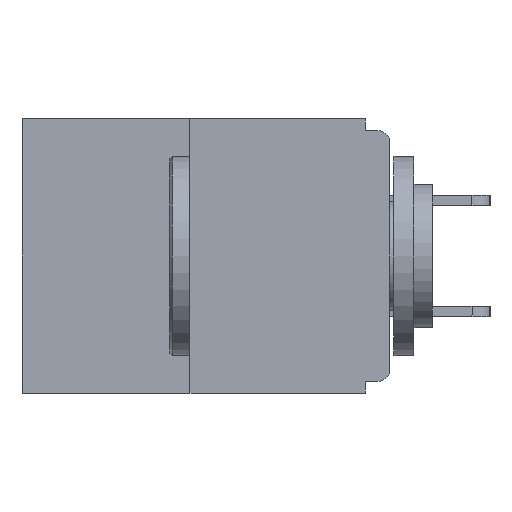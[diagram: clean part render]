
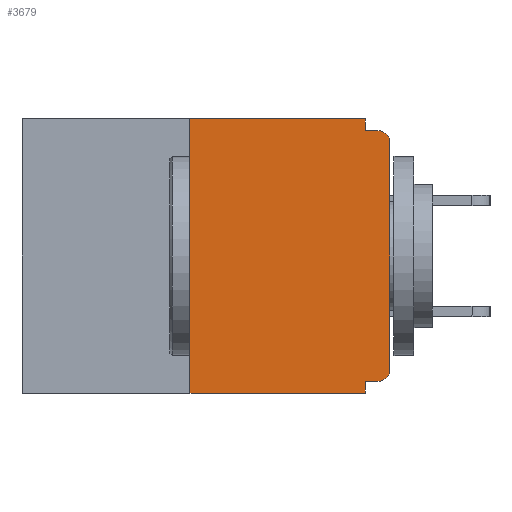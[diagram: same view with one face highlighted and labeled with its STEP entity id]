
A CAD part, left-side view. The second image highlights one B-rep face of the part: STEP entity #3679.
In plain terms, the highlighted planar face has unit normal (-1, 0, 0).
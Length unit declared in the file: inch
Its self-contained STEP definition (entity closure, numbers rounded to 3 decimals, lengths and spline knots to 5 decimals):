
#695 = CARTESIAN_POINT ( 'NONE',  ( 0., 0.031, 0. ) ) ;
#1478 = CARTESIAN_POINT ( 'NONE',  ( 0., 0.015, -0.313 ) ) ;
#1876 = ORIENTED_EDGE ( 'NONE', *, *, #5647, .F. ) ;
#1942 = CARTESIAN_POINT ( 'NONE',  ( 0., 0.46, 0. ) ) ;
#2201 = LINE ( 'NONE', #28071, #18874 ) ;
#2352 = CARTESIAN_POINT ( 'NONE',  ( 0., 0.015, -0.03 ) ) ;
#2702 = EDGE_CURVE ( 'NONE', #18080, #23388, #2201, .T. ) ;
#2946 = EDGE_LOOP ( 'NONE', ( #4588, #20163, #25656, #21828, #23723, #16641, #4883, #20448, #10286, #1876 ) ) ;
#3013 = CARTESIAN_POINT ( 'NONE',  ( 0., 0.031, -0.343 ) ) ;
#3679 = ADVANCED_FACE ( 'NONE', ( #6558 ), #10366, .F. ) ;
#3862 = CARTESIAN_POINT ( 'NONE',  ( 0., 0., -0.03 ) ) ;
#3897 = LINE ( 'NONE', #695, #11730 ) ;
#3924 = CARTESIAN_POINT ( 'NONE',  ( 0., 0.031, -0.015 ) ) ;
#4588 = ORIENTED_EDGE ( 'NONE', *, *, #27016, .F. ) ;
#4691 = DIRECTION ( 'NONE',  ( 0., 0., 1. ) ) ;
#4883 = ORIENTED_EDGE ( 'NONE', *, *, #10974, .T. ) ;
#5071 = LINE ( 'NONE', #19038, #19050 ) ;
#5340 = EDGE_CURVE ( 'NONE', #21721, #23388, #13786, .T. ) ;
#5486 = VERTEX_POINT ( 'NONE', #6380 ) ;
#5647 = EDGE_CURVE ( 'NONE', #19507, #10311, #3897, .T. ) ;
#6380 = CARTESIAN_POINT ( 'NONE',  ( 0., 0., -0.313 ) ) ;
#6484 = DIRECTION ( 'NONE',  ( 0., -1., 0. ) ) ;
#6558 = FACE_OUTER_BOUND ( 'NONE', #2946, .T. ) ;
#6775 = EDGE_CURVE ( 'NONE', #10311, #25107, #17444, .T. ) ;
#7209 = VECTOR ( 'NONE', #4691, 39.37008 ) ;
#7794 = DIRECTION ( 'NONE',  ( 0., 0., -1. ) ) ;
#7961 = LINE ( 'NONE', #1942, #25646 ) ;
#7981 = AXIS2_PLACEMENT_3D ( 'NONE', #2352, #28174, #24644 ) ;
#8359 = EDGE_CURVE ( 'NONE', #24460, #21721, #13274, .T. ) ;
#9212 = VERTEX_POINT ( 'NONE', #21654 ) ;
#9595 = CARTESIAN_POINT ( 'NONE',  ( 0., 0.031, 0. ) ) ;
#10286 = ORIENTED_EDGE ( 'NONE', *, *, #6775, .F. ) ;
#10311 = VERTEX_POINT ( 'NONE', #3924 ) ;
#10366 = PLANE ( 'NONE',  #26236 ) ;
#10974 = EDGE_CURVE ( 'NONE', #5486, #12482, #5071, .T. ) ;
#11730 = VECTOR ( 'NONE', #18114, 39.37008 ) ;
#12182 = CARTESIAN_POINT ( 'NONE',  ( 0., 0.46, 0. ) ) ;
#12482 = VERTEX_POINT ( 'NONE', #3862 ) ;
#12655 = DIRECTION ( 'NONE',  ( 0., 0., 1. ) ) ;
#13274 = LINE ( 'NONE', #15088, #23460 ) ;
#13507 = CARTESIAN_POINT ( 'NONE',  ( 0., 0.015, -0.328 ) ) ;
#13786 = LINE ( 'NONE', #20881, #24648 ) ;
#15088 = CARTESIAN_POINT ( 'NONE',  ( 0., 0., -0.328 ) ) ;
#15745 = VECTOR ( 'NONE', #25598, 39.37008 ) ;
#15865 = EDGE_CURVE ( 'NONE', #18080, #9212, #18818, .T. ) ;
#16104 = EDGE_CURVE ( 'NONE', #12482, #25107, #19480, .T. ) ;
#16430 = EDGE_CURVE ( 'NONE', #24460, #5486, #21475, .T. ) ;
#16641 = ORIENTED_EDGE ( 'NONE', *, *, #16430, .T. ) ;
#16699 = DIRECTION ( 'NONE',  ( -1., 0., 0. ) ) ;
#17444 = LINE ( 'NONE', #25686, #15745 ) ;
#18080 = VERTEX_POINT ( 'NONE', #27196 ) ;
#18114 = DIRECTION ( 'NONE',  ( 0., 0., -1. ) ) ;
#18667 = CARTESIAN_POINT ( 'NONE',  ( 0., 0.031, -0.328 ) ) ;
#18818 = LINE ( 'NONE', #19643, #7209 ) ;
#18874 = VECTOR ( 'NONE', #6484, 39.37008 ) ;
#19038 = CARTESIAN_POINT ( 'NONE',  ( 0., 0., 0. ) ) ;
#19050 = VECTOR ( 'NONE', #12655, 39.37008 ) ;
#19140 = AXIS2_PLACEMENT_3D ( 'NONE', #1478, #16699, #25392 ) ;
#19480 = CIRCLE ( 'NONE', #7981, 0.015 ) ;
#19492 = DIRECTION ( 'NONE',  ( 0., 1., 0. ) ) ;
#19507 = VERTEX_POINT ( 'NONE', #9595 ) ;
#19643 = CARTESIAN_POINT ( 'NONE',  ( 0., 0.25, 0. ) ) ;
#20163 = ORIENTED_EDGE ( 'NONE', *, *, #15865, .F. ) ;
#20448 = ORIENTED_EDGE ( 'NONE', *, *, #16104, .T. ) ;
#20881 = CARTESIAN_POINT ( 'NONE',  ( 0., 0.031, -0.343 ) ) ;
#21475 = CIRCLE ( 'NONE', #19140, 0.015 ) ;
#21654 = CARTESIAN_POINT ( 'NONE',  ( 0., 0.25, 0. ) ) ;
#21721 = VERTEX_POINT ( 'NONE', #18667 ) ;
#21828 = ORIENTED_EDGE ( 'NONE', *, *, #5340, .F. ) ;
#23388 = VERTEX_POINT ( 'NONE', #3013 ) ;
#23460 = VECTOR ( 'NONE', #19492, 39.37008 ) ;
#23723 = ORIENTED_EDGE ( 'NONE', *, *, #8359, .F. ) ;
#24460 = VERTEX_POINT ( 'NONE', #13507 ) ;
#24644 = DIRECTION ( 'NONE',  ( 0., 0., -1. ) ) ;
#24648 = VECTOR ( 'NONE', #27230, 39.37008 ) ;
#25107 = VERTEX_POINT ( 'NONE', #25331 ) ;
#25331 = CARTESIAN_POINT ( 'NONE',  ( 0., 0.015, -0.015 ) ) ;
#25392 = DIRECTION ( 'NONE',  ( 0., 0., -1. ) ) ;
#25598 = DIRECTION ( 'NONE',  ( 0., -1., 0. ) ) ;
#25646 = VECTOR ( 'NONE', #25660, 39.37008 ) ;
#25656 = ORIENTED_EDGE ( 'NONE', *, *, #2702, .T. ) ;
#25660 = DIRECTION ( 'NONE',  ( 0., -1., 0. ) ) ;
#25686 = CARTESIAN_POINT ( 'NONE',  ( 0., 0., -0.015 ) ) ;
#26236 = AXIS2_PLACEMENT_3D ( 'NONE', #12182, #27750, #7794 ) ;
#27016 = EDGE_CURVE ( 'NONE', #9212, #19507, #7961, .T. ) ;
#27196 = CARTESIAN_POINT ( 'NONE',  ( 0., 0.25, -0.343 ) ) ;
#27230 = DIRECTION ( 'NONE',  ( 0., 0., -1. ) ) ;
#27750 = DIRECTION ( 'NONE',  ( 1., 0., 0. ) ) ;
#28071 = CARTESIAN_POINT ( 'NONE',  ( 0., 0.46, -0.343 ) ) ;
#28174 = DIRECTION ( 'NONE',  ( -1., 0., 0. ) ) ;
